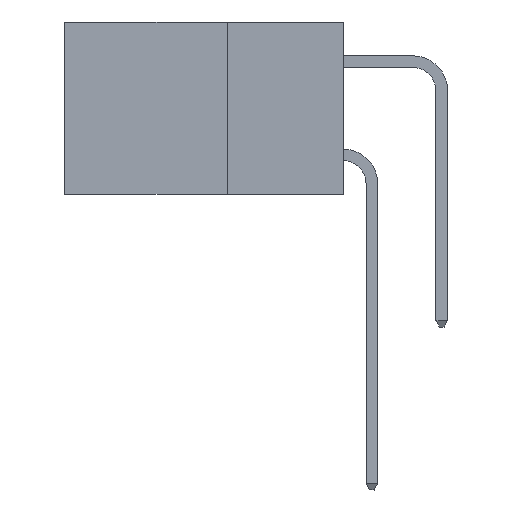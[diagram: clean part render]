
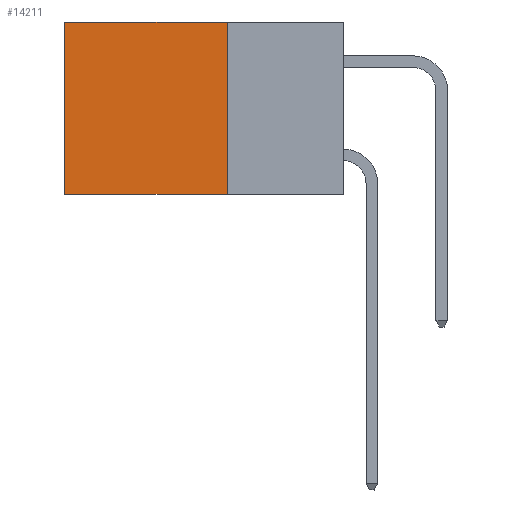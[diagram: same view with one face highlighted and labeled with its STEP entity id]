
A CAD part, left-side view. The second image highlights one B-rep face of the part: STEP entity #14211.
In plain terms, the highlighted planar face has unit normal (-1, 0, 0).
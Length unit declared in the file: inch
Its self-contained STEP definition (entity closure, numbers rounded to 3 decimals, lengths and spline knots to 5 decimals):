
#14 = LINE ( 'NONE', #1287, #1038 ) ;
#860 = AXIS2_PLACEMENT_3D ( 'NONE', #6797, #21162, #19510 ) ;
#1038 = VECTOR ( 'NONE', #14647, 39.37008 ) ;
#1287 = CARTESIAN_POINT ( 'NONE',  ( 0.298, 0.25, 0. ) ) ;
#1496 = VERTEX_POINT ( 'NONE', #3518 ) ;
#2003 = ORIENTED_EDGE ( 'NONE', *, *, #20460, .T. ) ;
#2262 = DIRECTION ( 'NONE',  ( 0., 1., 0. ) ) ;
#2434 = DIRECTION ( 'NONE',  ( 0., 0., -1. ) ) ;
#2779 = ORIENTED_EDGE ( 'NONE', *, *, #3952, .T. ) ;
#2905 = CARTESIAN_POINT ( 'NONE',  ( 0.298, 0.6, 0. ) ) ;
#3518 = CARTESIAN_POINT ( 'NONE',  ( 0.298, 0.6, -0.37 ) ) ;
#3952 = EDGE_CURVE ( 'NONE', #17826, #1496, #10372, .T. ) ;
#4112 = EDGE_CURVE ( 'NONE', #11142, #1496, #19205, .T. ) ;
#5174 = CARTESIAN_POINT ( 'NONE',  ( 0.298, 0.25, -0.37 ) ) ;
#6206 = DIRECTION ( 'NONE',  ( 0., 0., -1. ) ) ;
#6797 = CARTESIAN_POINT ( 'NONE',  ( 0.298, 0.25, 0. ) ) ;
#7491 = VECTOR ( 'NONE', #6206, 39.37008 ) ;
#7621 = VERTEX_POINT ( 'NONE', #20030 ) ;
#7916 = EDGE_LOOP ( 'NONE', ( #2779, #12935, #11094, #2003 ) ) ;
#8712 = EDGE_CURVE ( 'NONE', #7621, #11142, #8816, .T. ) ;
#8816 = LINE ( 'NONE', #17255, #14493 ) ;
#9656 = CARTESIAN_POINT ( 'NONE',  ( 0.298, 0.6, 0. ) ) ;
#10372 = LINE ( 'NONE', #2905, #7491 ) ;
#11094 = ORIENTED_EDGE ( 'NONE', *, *, #8712, .F. ) ;
#11142 = VERTEX_POINT ( 'NONE', #5174 ) ;
#12934 = VECTOR ( 'NONE', #2262, 39.37008 ) ;
#12935 = ORIENTED_EDGE ( 'NONE', *, *, #4112, .F. ) ;
#14211 = ADVANCED_FACE ( 'NONE', ( #20353 ), #15060, .F. ) ;
#14493 = VECTOR ( 'NONE', #2434, 39.37008 ) ;
#14647 = DIRECTION ( 'NONE',  ( 0., 1., 0. ) ) ;
#15060 = PLANE ( 'NONE',  #860 ) ;
#15323 = CARTESIAN_POINT ( 'NONE',  ( 0.298, 0.25, -0.37 ) ) ;
#17255 = CARTESIAN_POINT ( 'NONE',  ( 0.298, 0.25, 0. ) ) ;
#17826 = VERTEX_POINT ( 'NONE', #9656 ) ;
#19205 = LINE ( 'NONE', #15323, #12934 ) ;
#19510 = DIRECTION ( 'NONE',  ( 0., 0., -1. ) ) ;
#20030 = CARTESIAN_POINT ( 'NONE',  ( 0.298, 0.25, 0. ) ) ;
#20353 = FACE_OUTER_BOUND ( 'NONE', #7916, .T. ) ;
#20460 = EDGE_CURVE ( 'NONE', #7621, #17826, #14, .T. ) ;
#21162 = DIRECTION ( 'NONE',  ( 1., 0., 0. ) ) ;
